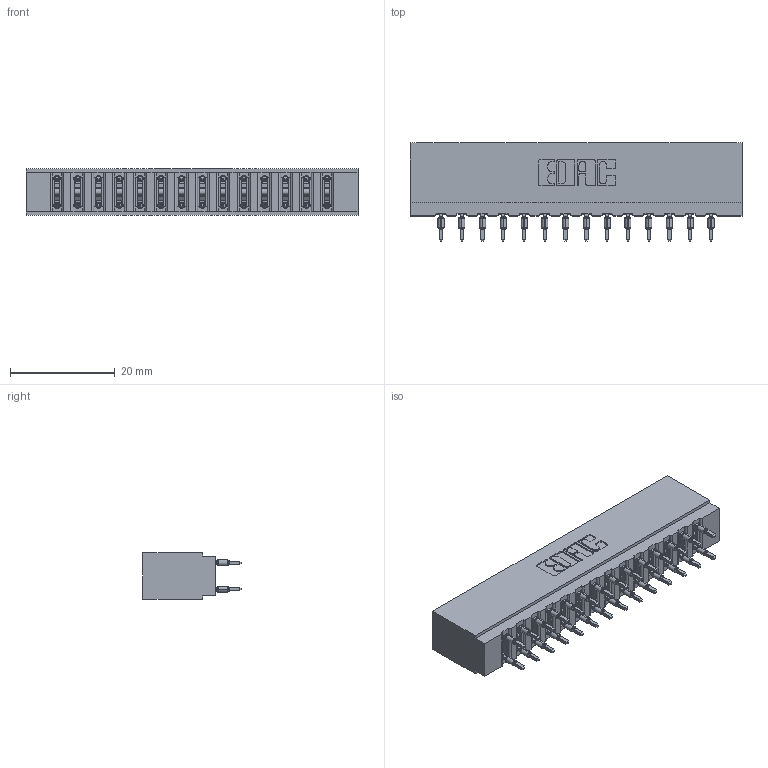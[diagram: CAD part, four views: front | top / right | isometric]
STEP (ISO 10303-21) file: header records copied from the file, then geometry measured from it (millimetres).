
FILE_DESCRIPTION (( 'STEP AP203' ), '1' );
FILE_NAME ('717-028-560-201.STEP', '2026-02-20T17:30:43', ( '' ), ( '' ), 'SwSTEP 2.0', 'SolidWorks 2023', '' );
FILE_SCHEMA (( 'CONFIG_CONTROL_DESIGN' ));
Length unit declared in the file: millimetre
Products named in the file (3): 717 Part_Insulator Option - 06; 745-292-001_560; 717-028-560-201
Assembly tree (29 placements, depth 2):
  717-028-560-201
    717 Part_Insulator Option - 06
    745-292-001_560  x28
Bounding box: 63.35 x 18.78 x 8.89 mm (x, y, z)
Volume: 5708.3 mm3; surface area: 8848.9 mm2
Topology: 29 solids, 29 shells, 2866 faces, 7839 edges, 4982 vertices
Faces by surface type: plane 1496, cylinder 642, bspline 560, torus 168
Entity records: 28108 total; most frequent: CARTESIAN_POINT 5391, ORIENTED_EDGE 4770, DIRECTION 4195, EDGE_CURVE 2385, LINE 2111, VECTOR 2111, VERTEX_POINT 1526, AXIS2_PLACEMENT_3D 1042
